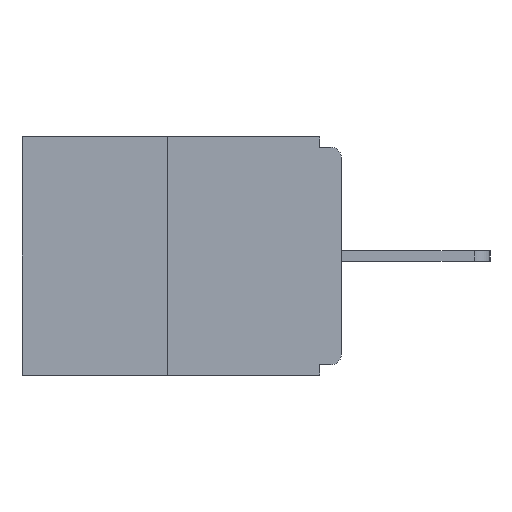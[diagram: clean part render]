
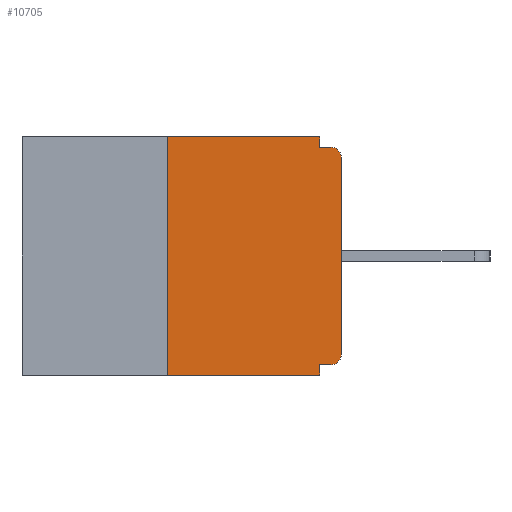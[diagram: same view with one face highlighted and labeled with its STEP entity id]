
A CAD part, left-side view. The second image highlights one B-rep face of the part: STEP entity #10705.
In plain terms, the highlighted planar face has unit normal (-1, 0, 0).
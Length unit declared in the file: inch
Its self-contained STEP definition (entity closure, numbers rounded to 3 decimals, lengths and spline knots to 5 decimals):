
#115 = CARTESIAN_POINT ( 'NONE',  ( 0., 0.46, 0. ) ) ;
#300 = VERTEX_POINT ( 'NONE', #14754 ) ;
#915 = CARTESIAN_POINT ( 'NONE',  ( 0., 0.46, 0. ) ) ;
#1787 = AXIS2_PLACEMENT_3D ( 'NONE', #5324, #18271, #5465 ) ;
#1835 = CARTESIAN_POINT ( 'NONE',  ( 0., 0.25, 0. ) ) ;
#2046 = EDGE_CURVE ( 'NONE', #12887, #23977, #15134, .T. ) ;
#2579 = DIRECTION ( 'NONE',  ( 1., 0., 0. ) ) ;
#3254 = ORIENTED_EDGE ( 'NONE', *, *, #12281, .T. ) ;
#3654 = LINE ( 'NONE', #12150, #5729 ) ;
#3666 = ORIENTED_EDGE ( 'NONE', *, *, #2046, .F. ) ;
#3705 = DIRECTION ( 'NONE',  ( 0., 0., -1. ) ) ;
#3758 = VERTEX_POINT ( 'NONE', #14621 ) ;
#3900 = EDGE_CURVE ( 'NONE', #14554, #300, #26434, .T. ) ;
#4093 = EDGE_CURVE ( 'NONE', #27441, #5766, #5512, .T. ) ;
#4432 = AXIS2_PLACEMENT_3D ( 'NONE', #915, #2579, #5204 ) ;
#4581 = DIRECTION ( 'NONE',  ( 0., 0., -1. ) ) ;
#4661 = PLANE ( 'NONE',  #4432 ) ;
#4723 = VECTOR ( 'NONE', #14580, 39.37008 ) ;
#5204 = DIRECTION ( 'NONE',  ( 0., 0., -1. ) ) ;
#5324 = CARTESIAN_POINT ( 'NONE',  ( 0., 0.015, -0.03 ) ) ;
#5465 = DIRECTION ( 'NONE',  ( 0., 0., -1. ) ) ;
#5512 = LINE ( 'NONE', #10370, #9791 ) ;
#5537 = CARTESIAN_POINT ( 'NONE',  ( 0., 0.031, 0. ) ) ;
#5729 = VECTOR ( 'NONE', #13827, 39.37008 ) ;
#5766 = VERTEX_POINT ( 'NONE', #7884 ) ;
#6219 = CIRCLE ( 'NONE', #1787, 0.015 ) ;
#6225 = EDGE_LOOP ( 'NONE', ( #13552, #3666, #6966, #22875, #7718, #25277, #11311, #3254, #26733, #23044 ) ) ;
#6229 = LINE ( 'NONE', #115, #4723 ) ;
#6966 = ORIENTED_EDGE ( 'NONE', *, *, #13640, .T. ) ;
#7612 = EDGE_CURVE ( 'NONE', #23977, #27441, #6229, .T. ) ;
#7718 = ORIENTED_EDGE ( 'NONE', *, *, #11298, .F. ) ;
#7884 = CARTESIAN_POINT ( 'NONE',  ( 0., 0.031, -0.015 ) ) ;
#8607 = VECTOR ( 'NONE', #25979, 39.37008 ) ;
#8737 = CARTESIAN_POINT ( 'NONE',  ( 0., 0.25, 0. ) ) ;
#8862 = DIRECTION ( 'NONE',  ( 0., 0., -1. ) ) ;
#9791 = VECTOR ( 'NONE', #3705, 39.37008 ) ;
#10066 = DIRECTION ( 'NONE',  ( 0., -1., 0. ) ) ;
#10370 = CARTESIAN_POINT ( 'NONE',  ( 0., 0.031, 0. ) ) ;
#10371 = LINE ( 'NONE', #14423, #26404 ) ;
#10704 = VECTOR ( 'NONE', #16188, 39.37008 ) ;
#10705 = ADVANCED_FACE ( 'NONE', ( #19954 ), #4661, .F. ) ;
#11298 = EDGE_CURVE ( 'NONE', #14554, #23267, #3654, .T. ) ;
#11311 = ORIENTED_EDGE ( 'NONE', *, *, #24887, .T. ) ;
#11605 = EDGE_CURVE ( 'NONE', #23267, #3758, #23598, .T. ) ;
#11635 = CARTESIAN_POINT ( 'NONE',  ( 0., 0.015, -0.313 ) ) ;
#11870 = LINE ( 'NONE', #22439, #10704 ) ;
#12150 = CARTESIAN_POINT ( 'NONE',  ( 0., 0., -0.328 ) ) ;
#12164 = LINE ( 'NONE', #20638, #27170 ) ;
#12281 = EDGE_CURVE ( 'NONE', #22544, #25935, #6219, .T. ) ;
#12668 = AXIS2_PLACEMENT_3D ( 'NONE', #11635, #18169, #4581 ) ;
#12887 = VERTEX_POINT ( 'NONE', #25595 ) ;
#13552 = ORIENTED_EDGE ( 'NONE', *, *, #7612, .F. ) ;
#13593 = EDGE_CURVE ( 'NONE', #5766, #25935, #11870, .T. ) ;
#13640 = EDGE_CURVE ( 'NONE', #12887, #3758, #12164, .T. ) ;
#13827 = DIRECTION ( 'NONE',  ( 0., 1., 0. ) ) ;
#14423 = CARTESIAN_POINT ( 'NONE',  ( 0., 0., 0. ) ) ;
#14554 = VERTEX_POINT ( 'NONE', #16671 ) ;
#14580 = DIRECTION ( 'NONE',  ( 0., -1., 0. ) ) ;
#14621 = CARTESIAN_POINT ( 'NONE',  ( 0., 0.031, -0.343 ) ) ;
#14754 = CARTESIAN_POINT ( 'NONE',  ( 0., 0., -0.313 ) ) ;
#15134 = LINE ( 'NONE', #8737, #8607 ) ;
#16188 = DIRECTION ( 'NONE',  ( 0., -1., 0. ) ) ;
#16671 = CARTESIAN_POINT ( 'NONE',  ( 0., 0.015, -0.328 ) ) ;
#16846 = VECTOR ( 'NONE', #8862, 39.37008 ) ;
#18169 = DIRECTION ( 'NONE',  ( -1., 0., 0. ) ) ;
#18271 = DIRECTION ( 'NONE',  ( -1., 0., 0. ) ) ;
#19954 = FACE_OUTER_BOUND ( 'NONE', #6225, .T. ) ;
#20638 = CARTESIAN_POINT ( 'NONE',  ( 0., 0.46, -0.343 ) ) ;
#20977 = CARTESIAN_POINT ( 'NONE',  ( 0., 0.031, -0.328 ) ) ;
#21184 = CARTESIAN_POINT ( 'NONE',  ( 0., 0., -0.03 ) ) ;
#21939 = CARTESIAN_POINT ( 'NONE',  ( 0., 0.015, -0.015 ) ) ;
#22439 = CARTESIAN_POINT ( 'NONE',  ( 0., 0., -0.015 ) ) ;
#22544 = VERTEX_POINT ( 'NONE', #21184 ) ;
#22875 = ORIENTED_EDGE ( 'NONE', *, *, #11605, .F. ) ;
#22896 = DIRECTION ( 'NONE',  ( 0., 0., 1. ) ) ;
#23044 = ORIENTED_EDGE ( 'NONE', *, *, #4093, .F. ) ;
#23267 = VERTEX_POINT ( 'NONE', #20977 ) ;
#23598 = LINE ( 'NONE', #23731, #16846 ) ;
#23731 = CARTESIAN_POINT ( 'NONE',  ( 0., 0.031, -0.343 ) ) ;
#23977 = VERTEX_POINT ( 'NONE', #1835 ) ;
#24887 = EDGE_CURVE ( 'NONE', #300, #22544, #10371, .T. ) ;
#25277 = ORIENTED_EDGE ( 'NONE', *, *, #3900, .T. ) ;
#25595 = CARTESIAN_POINT ( 'NONE',  ( 0., 0.25, -0.343 ) ) ;
#25935 = VERTEX_POINT ( 'NONE', #21939 ) ;
#25979 = DIRECTION ( 'NONE',  ( 0., 0., 1. ) ) ;
#26404 = VECTOR ( 'NONE', #22896, 39.37008 ) ;
#26434 = CIRCLE ( 'NONE', #12668, 0.015 ) ;
#26733 = ORIENTED_EDGE ( 'NONE', *, *, #13593, .F. ) ;
#27170 = VECTOR ( 'NONE', #10066, 39.37008 ) ;
#27441 = VERTEX_POINT ( 'NONE', #5537 ) ;
